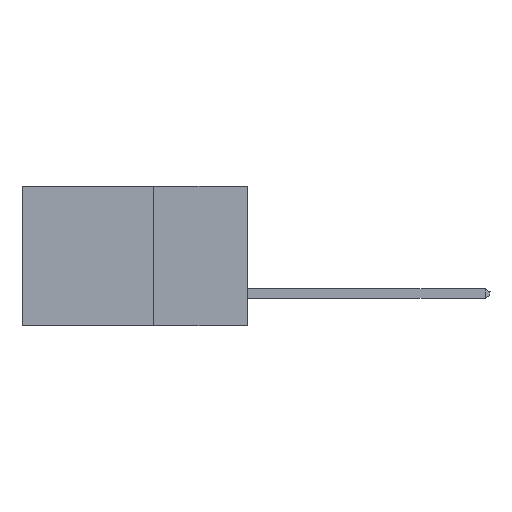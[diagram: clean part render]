
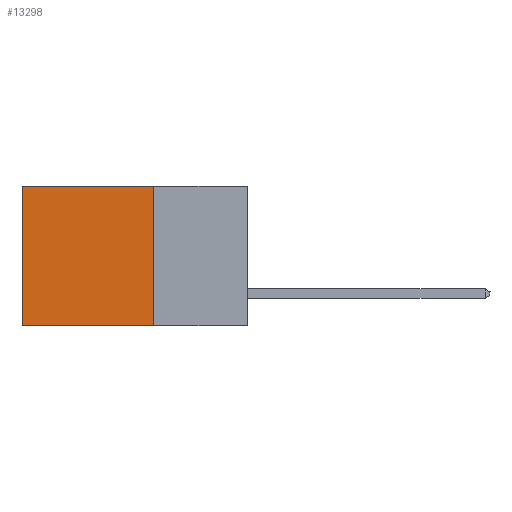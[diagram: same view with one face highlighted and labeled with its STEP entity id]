
A CAD part, left-side view. The second image highlights one B-rep face of the part: STEP entity #13298.
In plain terms, the highlighted planar face has unit normal (-1, 0, 0).
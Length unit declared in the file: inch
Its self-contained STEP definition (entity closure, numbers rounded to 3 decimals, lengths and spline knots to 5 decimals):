
#385 = LINE ( 'NONE', #3464, #834 ) ;
#834 = VECTOR ( 'NONE', #6208, 39.37008 ) ;
#1319 = CARTESIAN_POINT ( 'NONE',  ( 0.2615, 0.25, -0.37 ) ) ;
#1323 = VECTOR ( 'NONE', #7865, 39.37008 ) ;
#2046 = EDGE_CURVE ( 'NONE', #10489, #4669, #13786, .T. ) ;
#2680 = DIRECTION ( 'NONE',  ( 0., 1., 0. ) ) ;
#2888 = EDGE_CURVE ( 'NONE', #5703, #4669, #385, .T. ) ;
#3175 = EDGE_LOOP ( 'NONE', ( #4266, #11792, #14793, #8485 ) ) ;
#3464 = CARTESIAN_POINT ( 'NONE',  ( 0.2615, 0.6, -0.37 ) ) ;
#4266 = ORIENTED_EDGE ( 'NONE', *, *, #2888, .T. ) ;
#4662 = LINE ( 'NONE', #7393, #4939 ) ;
#4669 = VERTEX_POINT ( 'NONE', #15820 ) ;
#4939 = VECTOR ( 'NONE', #16868, 39.37008 ) ;
#5703 = VERTEX_POINT ( 'NONE', #9055 ) ;
#6208 = DIRECTION ( 'NONE',  ( 0., 0., -1. ) ) ;
#7393 = CARTESIAN_POINT ( 'NONE',  ( 0.2615, 0.25, 0. ) ) ;
#7686 = DIRECTION ( 'NONE',  ( 0., 0., -1. ) ) ;
#7865 = DIRECTION ( 'NONE',  ( 0., 0., -1. ) ) ;
#8485 = ORIENTED_EDGE ( 'NONE', *, *, #9434, .T. ) ;
#8790 = DIRECTION ( 'NONE',  ( 1., 0., 0. ) ) ;
#9055 = CARTESIAN_POINT ( 'NONE',  ( 0.2615, 0.6, 0. ) ) ;
#9434 = EDGE_CURVE ( 'NONE', #15192, #5703, #4662, .T. ) ;
#10420 = PLANE ( 'NONE',  #14880 ) ;
#10489 = VERTEX_POINT ( 'NONE', #12152 ) ;
#11126 = VECTOR ( 'NONE', #2680, 39.37008 ) ;
#11792 = ORIENTED_EDGE ( 'NONE', *, *, #2046, .F. ) ;
#12152 = CARTESIAN_POINT ( 'NONE',  ( 0.2615, 0.25, -0.37 ) ) ;
#13298 = ADVANCED_FACE ( 'NONE', ( #14693 ), #10420, .F. ) ;
#13786 = LINE ( 'NONE', #16414, #11126 ) ;
#14484 = CARTESIAN_POINT ( 'NONE',  ( 0.2615, 0.25, 0. ) ) ;
#14693 = FACE_OUTER_BOUND ( 'NONE', #3175, .T. ) ;
#14793 = ORIENTED_EDGE ( 'NONE', *, *, #17396, .F. ) ;
#14880 = AXIS2_PLACEMENT_3D ( 'NONE', #17066, #8790, #7686 ) ;
#15192 = VERTEX_POINT ( 'NONE', #14484 ) ;
#15820 = CARTESIAN_POINT ( 'NONE',  ( 0.2615, 0.6, -0.37 ) ) ;
#16222 = LINE ( 'NONE', #1319, #1323 ) ;
#16414 = CARTESIAN_POINT ( 'NONE',  ( 0.2615, 0.25, -0.37 ) ) ;
#16868 = DIRECTION ( 'NONE',  ( 0., 1., 0. ) ) ;
#17066 = CARTESIAN_POINT ( 'NONE',  ( 0.2615, 0.25, -0.37 ) ) ;
#17396 = EDGE_CURVE ( 'NONE', #15192, #10489, #16222, .T. ) ;
